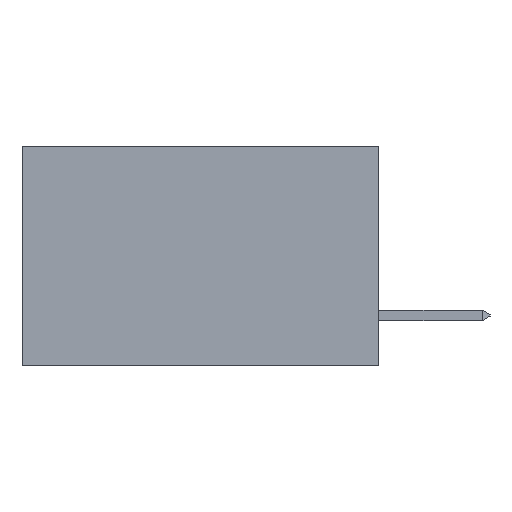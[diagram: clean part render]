
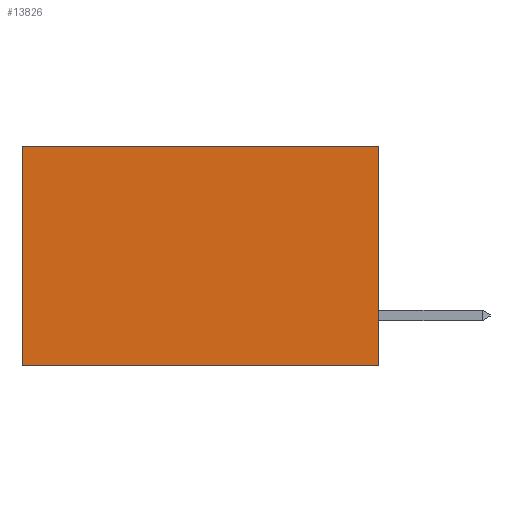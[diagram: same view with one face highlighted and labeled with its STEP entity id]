
A CAD part, left-side view. The second image highlights one B-rep face of the part: STEP entity #13826.
In plain terms, the highlighted planar face has unit normal (-1, 0, 0).
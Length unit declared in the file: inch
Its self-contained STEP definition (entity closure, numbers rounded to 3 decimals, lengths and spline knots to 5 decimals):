
#59 = VERTEX_POINT ( 'NONE', #2308 ) ;
#559 = CARTESIAN_POINT ( 'NONE',  ( 0.298, 0., 0. ) ) ;
#574 = DIRECTION ( 'NONE',  ( 0., 0., -1. ) ) ;
#1343 = CARTESIAN_POINT ( 'NONE',  ( 0.298, 0.6, 0. ) ) ;
#2158 = VECTOR ( 'NONE', #574, 39.37008 ) ;
#2308 = CARTESIAN_POINT ( 'NONE',  ( 0.298, 0., -0.37 ) ) ;
#3017 = LINE ( 'NONE', #559, #14809 ) ;
#3496 = ORIENTED_EDGE ( 'NONE', *, *, #5121, .T. ) ;
#4124 = DIRECTION ( 'NONE',  ( 0., 0., -1. ) ) ;
#4224 = ORIENTED_EDGE ( 'NONE', *, *, #10607, .T. ) ;
#4996 = VERTEX_POINT ( 'NONE', #9612 ) ;
#5121 = EDGE_CURVE ( 'NONE', #4996, #10250, #3017, .T. ) ;
#5347 = FACE_OUTER_BOUND ( 'NONE', #8294, .T. ) ;
#5612 = CARTESIAN_POINT ( 'NONE',  ( 0.298, 0., 0. ) ) ;
#5642 = AXIS2_PLACEMENT_3D ( 'NONE', #9996, #11150, #4124 ) ;
#5788 = CARTESIAN_POINT ( 'NONE',  ( 0.298, 0.6, -0.37 ) ) ;
#7258 = VERTEX_POINT ( 'NONE', #5788 ) ;
#7513 = DIRECTION ( 'NONE',  ( 0., 0., -1. ) ) ;
#8294 = EDGE_LOOP ( 'NONE', ( #4224, #11589, #12038, #3496 ) ) ;
#8366 = EDGE_CURVE ( 'NONE', #4996, #59, #11624, .T. ) ;
#8503 = DIRECTION ( 'NONE',  ( 0., 1., 0. ) ) ;
#8874 = PLANE ( 'NONE',  #5642 ) ;
#9037 = DIRECTION ( 'NONE',  ( 0., 1., 0. ) ) ;
#9281 = CARTESIAN_POINT ( 'NONE',  ( 0.298, 0.6, 0. ) ) ;
#9612 = CARTESIAN_POINT ( 'NONE',  ( 0.298, 0., 0. ) ) ;
#9996 = CARTESIAN_POINT ( 'NONE',  ( 0.298, 0., 0. ) ) ;
#10250 = VERTEX_POINT ( 'NONE', #9281 ) ;
#10607 = EDGE_CURVE ( 'NONE', #10250, #7258, #11893, .T. ) ;
#11150 = DIRECTION ( 'NONE',  ( 1., 0., 0. ) ) ;
#11589 = ORIENTED_EDGE ( 'NONE', *, *, #14257, .F. ) ;
#11624 = LINE ( 'NONE', #5612, #2158 ) ;
#11864 = LINE ( 'NONE', #15045, #12208 ) ;
#11893 = LINE ( 'NONE', #1343, #14335 ) ;
#12038 = ORIENTED_EDGE ( 'NONE', *, *, #8366, .F. ) ;
#12208 = VECTOR ( 'NONE', #8503, 39.37008 ) ;
#13826 = ADVANCED_FACE ( 'NONE', ( #5347 ), #8874, .F. ) ;
#14257 = EDGE_CURVE ( 'NONE', #59, #7258, #11864, .T. ) ;
#14335 = VECTOR ( 'NONE', #7513, 39.37008 ) ;
#14809 = VECTOR ( 'NONE', #9037, 39.37008 ) ;
#15045 = CARTESIAN_POINT ( 'NONE',  ( 0.298, 0., -0.37 ) ) ;
